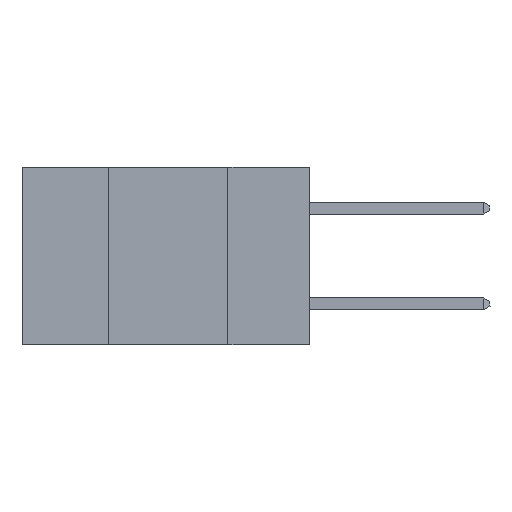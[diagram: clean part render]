
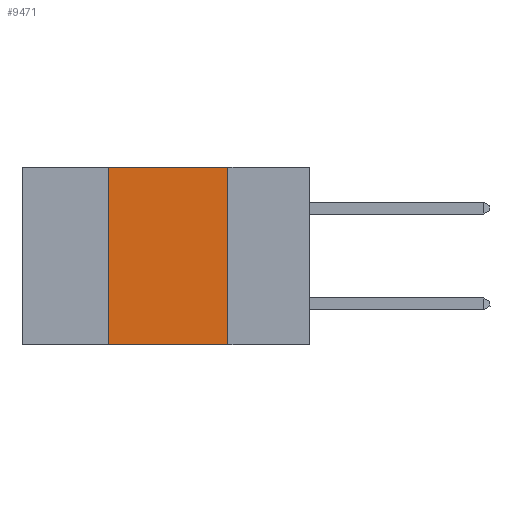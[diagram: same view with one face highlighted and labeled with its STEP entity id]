
A CAD part, left-side view. The second image highlights one B-rep face of the part: STEP entity #9471.
In plain terms, the highlighted planar face has unit normal (-1, 0, 0).
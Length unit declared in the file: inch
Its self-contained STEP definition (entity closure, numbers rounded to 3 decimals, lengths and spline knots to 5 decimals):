
#15 = ORIENTED_EDGE ( 'NONE', *, *, #6226, .T. ) ;
#165 = DIRECTION ( 'NONE',  ( 0., -1., 0. ) ) ;
#422 = VERTEX_POINT ( 'NONE', #2850 ) ;
#519 = EDGE_LOOP ( 'NONE', ( #5827, #4446, #10189, #15 ) ) ;
#638 = CARTESIAN_POINT ( 'NONE',  ( 0., 0.17, 0. ) ) ;
#774 = DIRECTION ( 'NONE',  ( 0., 0., -1. ) ) ;
#844 = CARTESIAN_POINT ( 'NONE',  ( 0., 0.42, 0. ) ) ;
#870 = CARTESIAN_POINT ( 'NONE',  ( 0., 0.42, 0. ) ) ;
#991 = VECTOR ( 'NONE', #165, 39.37008 ) ;
#1595 = AXIS2_PLACEMENT_3D ( 'NONE', #3961, #4060, #774 ) ;
#1663 = PLANE ( 'NONE',  #1595 ) ;
#2337 = EDGE_CURVE ( 'NONE', #6460, #422, #3482, .T. ) ;
#2850 = CARTESIAN_POINT ( 'NONE',  ( 0., 0.17, 0. ) ) ;
#2947 = EDGE_CURVE ( 'NONE', #10248, #6460, #8254, .T. ) ;
#3004 = DIRECTION ( 'NONE',  ( 0., -1., 0. ) ) ;
#3174 = FACE_OUTER_BOUND ( 'NONE', #519, .T. ) ;
#3180 = VECTOR ( 'NONE', #3004, 39.37008 ) ;
#3227 = LINE ( 'NONE', #638, #4592 ) ;
#3363 = EDGE_CURVE ( 'NONE', #422, #9881, #3227, .T. ) ;
#3482 = LINE ( 'NONE', #5860, #991 ) ;
#3961 = CARTESIAN_POINT ( 'NONE',  ( 0., 0.6, 0. ) ) ;
#4060 = DIRECTION ( 'NONE',  ( 1., 0., 0. ) ) ;
#4297 = LINE ( 'NONE', #7891, #3180 ) ;
#4328 = CARTESIAN_POINT ( 'NONE',  ( 0., 0.42, -0.37 ) ) ;
#4446 = ORIENTED_EDGE ( 'NONE', *, *, #2337, .F. ) ;
#4592 = VECTOR ( 'NONE', #9362, 39.37008 ) ;
#4902 = DIRECTION ( 'NONE',  ( 0., 0., 1. ) ) ;
#5827 = ORIENTED_EDGE ( 'NONE', *, *, #3363, .F. ) ;
#5860 = CARTESIAN_POINT ( 'NONE',  ( 0., 0.6, 0. ) ) ;
#6129 = VECTOR ( 'NONE', #4902, 39.37008 ) ;
#6226 = EDGE_CURVE ( 'NONE', #10248, #9881, #4297, .T. ) ;
#6460 = VERTEX_POINT ( 'NONE', #870 ) ;
#7891 = CARTESIAN_POINT ( 'NONE',  ( 0., 0.6, -0.37 ) ) ;
#8254 = LINE ( 'NONE', #844, #6129 ) ;
#9190 = CARTESIAN_POINT ( 'NONE',  ( 0., 0.17, -0.37 ) ) ;
#9362 = DIRECTION ( 'NONE',  ( 0., 0., -1. ) ) ;
#9471 = ADVANCED_FACE ( 'NONE', ( #3174 ), #1663, .F. ) ;
#9881 = VERTEX_POINT ( 'NONE', #9190 ) ;
#10189 = ORIENTED_EDGE ( 'NONE', *, *, #2947, .F. ) ;
#10248 = VERTEX_POINT ( 'NONE', #4328 ) ;
